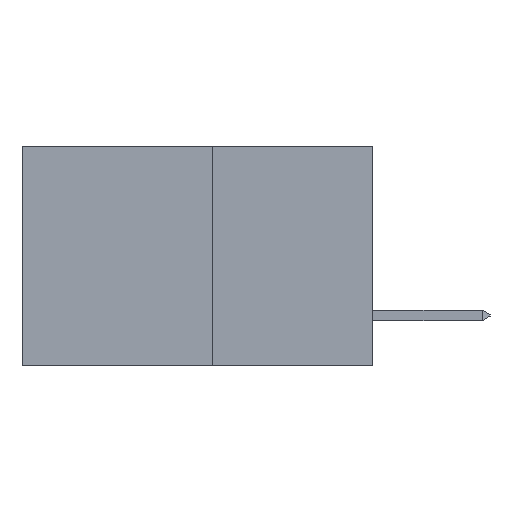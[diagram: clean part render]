
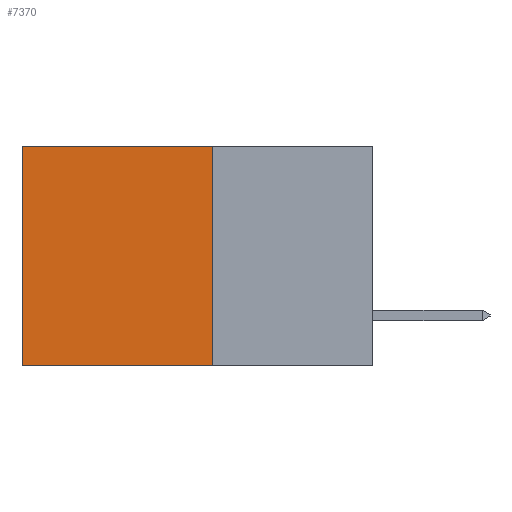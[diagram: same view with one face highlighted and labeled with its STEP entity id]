
A CAD part, left-side view. The second image highlights one B-rep face of the part: STEP entity #7370.
In plain terms, the highlighted planar face has unit normal (-1, 0, 0).
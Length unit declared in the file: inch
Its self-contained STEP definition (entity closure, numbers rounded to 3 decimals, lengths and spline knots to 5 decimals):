
#247 = CARTESIAN_POINT ( 'NONE',  ( 0.277, 0.27, -0.37 ) ) ;
#252 = VECTOR ( 'NONE', #24372, 39.37008 ) ;
#1145 = CARTESIAN_POINT ( 'NONE',  ( 0.277, 0.27, -0.37 ) ) ;
#1878 = LINE ( 'NONE', #6170, #24769 ) ;
#2579 = DIRECTION ( 'NONE',  ( 0., 0., -1. ) ) ;
#4004 = VECTOR ( 'NONE', #9757, 39.37008 ) ;
#4119 = EDGE_CURVE ( 'NONE', #6017, #7848, #23180, .T. ) ;
#5061 = CARTESIAN_POINT ( 'NONE',  ( 0.277, 0.59, -0.37 ) ) ;
#5410 = VERTEX_POINT ( 'NONE', #7353 ) ;
#6011 = VERTEX_POINT ( 'NONE', #5061 ) ;
#6017 = VERTEX_POINT ( 'NONE', #7226 ) ;
#6081 = VECTOR ( 'NONE', #19435, 39.37008 ) ;
#6170 = CARTESIAN_POINT ( 'NONE',  ( 0.277, 0.59, -0.37 ) ) ;
#7226 = CARTESIAN_POINT ( 'NONE',  ( 0.277, 0.27, 0. ) ) ;
#7353 = CARTESIAN_POINT ( 'NONE',  ( 0.277, 0.59, 0. ) ) ;
#7370 = ADVANCED_FACE ( 'NONE', ( #22313 ), #21941, .F. ) ;
#7848 = VERTEX_POINT ( 'NONE', #247 ) ;
#8333 = DIRECTION ( 'NONE',  ( 0., 0., -1. ) ) ;
#9757 = DIRECTION ( 'NONE',  ( 0., 1., 0. ) ) ;
#10389 = LINE ( 'NONE', #1145, #4004 ) ;
#10546 = ORIENTED_EDGE ( 'NONE', *, *, #4119, .F. ) ;
#10737 = CARTESIAN_POINT ( 'NONE',  ( 0.277, 0.27, 0. ) ) ;
#13275 = ORIENTED_EDGE ( 'NONE', *, *, #17180, .F. ) ;
#15541 = DIRECTION ( 'NONE',  ( 1., 0., 0. ) ) ;
#15669 = ORIENTED_EDGE ( 'NONE', *, *, #16233, .T. ) ;
#16233 = EDGE_CURVE ( 'NONE', #6017, #5410, #23970, .T. ) ;
#17180 = EDGE_CURVE ( 'NONE', #7848, #6011, #10389, .T. ) ;
#19435 = DIRECTION ( 'NONE',  ( 0., 1., 0. ) ) ;
#20030 = CARTESIAN_POINT ( 'NONE',  ( 0.277, 0.27, -0.37 ) ) ;
#21941 = PLANE ( 'NONE',  #23057 ) ;
#22013 = EDGE_CURVE ( 'NONE', #5410, #6011, #1878, .T. ) ;
#22313 = FACE_OUTER_BOUND ( 'NONE', #27265, .T. ) ;
#23057 = AXIS2_PLACEMENT_3D ( 'NONE', #26206, #15541, #2579 ) ;
#23180 = LINE ( 'NONE', #20030, #252 ) ;
#23970 = LINE ( 'NONE', #10737, #6081 ) ;
#24372 = DIRECTION ( 'NONE',  ( 0., 0., -1. ) ) ;
#24769 = VECTOR ( 'NONE', #8333, 39.37008 ) ;
#25889 = ORIENTED_EDGE ( 'NONE', *, *, #22013, .T. ) ;
#26206 = CARTESIAN_POINT ( 'NONE',  ( 0.277, 0.27, -0.37 ) ) ;
#27265 = EDGE_LOOP ( 'NONE', ( #25889, #13275, #10546, #15669 ) ) ;
